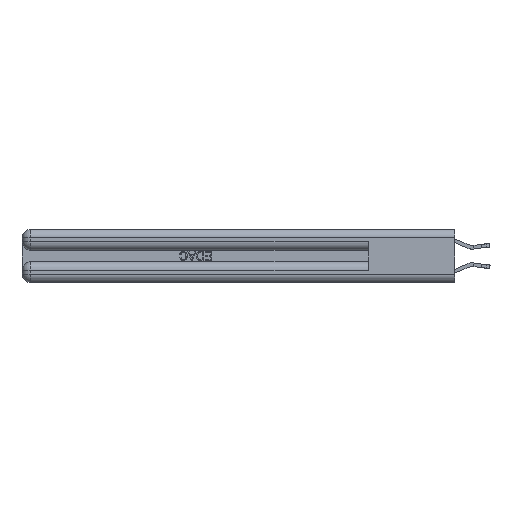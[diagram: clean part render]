
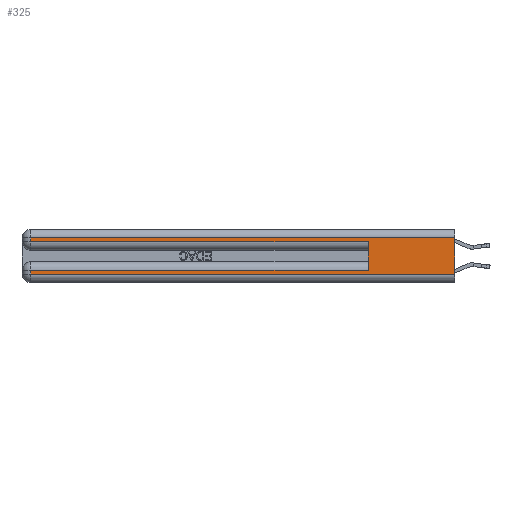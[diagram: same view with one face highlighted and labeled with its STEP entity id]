
A CAD part, left-side view. The second image highlights one B-rep face of the part: STEP entity #325.
In plain terms, the highlighted planar face has unit normal (-1, 0, 0).
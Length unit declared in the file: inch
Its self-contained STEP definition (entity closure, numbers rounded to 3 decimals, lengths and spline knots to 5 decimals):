
#17 = CARTESIAN_POINT ( 'NONE',  ( 0., 2.94, 0.085 ) ) ;
#325 = ADVANCED_FACE ( 'NONE', ( #17375 ), #10696, .F. ) ;
#335 = CARTESIAN_POINT ( 'NONE',  ( 0., 2.94, 0.285 ) ) ;
#1015 = EDGE_LOOP ( 'NONE', ( #27941, #22565, #4123, #26531, #24649, #1185, #6772, #17816 ) ) ;
#1168 = CARTESIAN_POINT ( 'NONE',  ( 0., 2.94, 0.37 ) ) ;
#1185 = ORIENTED_EDGE ( 'NONE', *, *, #25281, .T. ) ;
#1604 = CARTESIAN_POINT ( 'NONE',  ( 0., 0., 0.06 ) ) ;
#1729 = CARTESIAN_POINT ( 'NONE',  ( 0., 0., 0.31 ) ) ;
#3214 = EDGE_CURVE ( 'NONE', #27046, #27026, #27823, .T. ) ;
#4123 = ORIENTED_EDGE ( 'NONE', *, *, #29587, .T. ) ;
#4494 = VERTEX_POINT ( 'NONE', #27971 ) ;
#5132 = VECTOR ( 'NONE', #17609, 39.37008 ) ;
#5583 = EDGE_CURVE ( 'NONE', #21822, #4494, #6006, .T. ) ;
#6006 = LINE ( 'NONE', #1729, #16646 ) ;
#6173 = CARTESIAN_POINT ( 'NONE',  ( 0., 0., 0.285 ) ) ;
#6772 = ORIENTED_EDGE ( 'NONE', *, *, #12108, .T. ) ;
#7667 = LINE ( 'NONE', #13862, #24951 ) ;
#8050 = VECTOR ( 'NONE', #26826, 39.37008 ) ;
#8410 = DIRECTION ( 'NONE',  ( 1., 0., 0. ) ) ;
#8516 = CARTESIAN_POINT ( 'NONE',  ( 0., 0., 0.37 ) ) ;
#8801 = LINE ( 'NONE', #1168, #5132 ) ;
#8876 = DIRECTION ( 'NONE',  ( 0., -1., 0. ) ) ;
#8949 = VERTEX_POINT ( 'NONE', #23475 ) ;
#9177 = CARTESIAN_POINT ( 'NONE',  ( 0., 0.6, 0.145 ) ) ;
#10412 = CARTESIAN_POINT ( 'NONE',  ( 0., 0., 0.085 ) ) ;
#10696 = PLANE ( 'NONE',  #25810 ) ;
#11156 = VECTOR ( 'NONE', #14188, 39.37008 ) ;
#12108 = EDGE_CURVE ( 'NONE', #26962, #8949, #8801, .T. ) ;
#12229 = CARTESIAN_POINT ( 'NONE',  ( 0., 0., 0.31 ) ) ;
#12428 = EDGE_CURVE ( 'NONE', #21822, #18308, #7667, .T. ) ;
#13729 = DIRECTION ( 'NONE',  ( 0., 1., 0. ) ) ;
#13862 = CARTESIAN_POINT ( 'NONE',  ( 0., 0., 0.37 ) ) ;
#14188 = DIRECTION ( 'NONE',  ( 0., 0., 1. ) ) ;
#14235 = VECTOR ( 'NONE', #27121, 39.37008 ) ;
#15751 = DIRECTION ( 'NONE',  ( 0., 0., -1. ) ) ;
#16646 = VECTOR ( 'NONE', #13729, 39.37008 ) ;
#17375 = FACE_OUTER_BOUND ( 'NONE', #1015, .T. ) ;
#17609 = DIRECTION ( 'NONE',  ( 0., 0., -1. ) ) ;
#17816 = ORIENTED_EDGE ( 'NONE', *, *, #19616, .T. ) ;
#17860 = CARTESIAN_POINT ( 'NONE',  ( 0., 0.6, 0.085 ) ) ;
#18063 = EDGE_CURVE ( 'NONE', #24767, #27026, #29871, .T. ) ;
#18308 = VERTEX_POINT ( 'NONE', #20994 ) ;
#18718 = LINE ( 'NONE', #1604, #28209 ) ;
#19019 = VECTOR ( 'NONE', #15751, 39.37008 ) ;
#19130 = LINE ( 'NONE', #10412, #8050 ) ;
#19399 = LINE ( 'NONE', #20140, #19019 ) ;
#19616 = EDGE_CURVE ( 'NONE', #8949, #18308, #18718, .T. ) ;
#19984 = DIRECTION ( 'NONE',  ( 0., 0., -1. ) ) ;
#20140 = CARTESIAN_POINT ( 'NONE',  ( 0., 2.94, 0.37 ) ) ;
#20994 = CARTESIAN_POINT ( 'NONE',  ( 0., 0., 0.06 ) ) ;
#21669 = CARTESIAN_POINT ( 'NONE',  ( 0., 0.6, 0.285 ) ) ;
#21822 = VERTEX_POINT ( 'NONE', #12229 ) ;
#22565 = ORIENTED_EDGE ( 'NONE', *, *, #5583, .T. ) ;
#23475 = CARTESIAN_POINT ( 'NONE',  ( 0., 2.94, 0.06 ) ) ;
#24649 = ORIENTED_EDGE ( 'NONE', *, *, #18063, .F. ) ;
#24767 = VERTEX_POINT ( 'NONE', #17860 ) ;
#24951 = VECTOR ( 'NONE', #27838, 39.37008 ) ;
#25281 = EDGE_CURVE ( 'NONE', #24767, #26962, #19130, .T. ) ;
#25810 = AXIS2_PLACEMENT_3D ( 'NONE', #8516, #8410, #19984 ) ;
#26531 = ORIENTED_EDGE ( 'NONE', *, *, #3214, .T. ) ;
#26826 = DIRECTION ( 'NONE',  ( 0., 1., 0. ) ) ;
#26962 = VERTEX_POINT ( 'NONE', #17 ) ;
#27026 = VERTEX_POINT ( 'NONE', #21669 ) ;
#27046 = VERTEX_POINT ( 'NONE', #335 ) ;
#27121 = DIRECTION ( 'NONE',  ( 0., -1., 0. ) ) ;
#27823 = LINE ( 'NONE', #6173, #14235 ) ;
#27838 = DIRECTION ( 'NONE',  ( 0., 0., -1. ) ) ;
#27941 = ORIENTED_EDGE ( 'NONE', *, *, #12428, .F. ) ;
#27971 = CARTESIAN_POINT ( 'NONE',  ( 0., 2.94, 0.31 ) ) ;
#28209 = VECTOR ( 'NONE', #8876, 39.37008 ) ;
#29587 = EDGE_CURVE ( 'NONE', #4494, #27046, #19399, .T. ) ;
#29871 = LINE ( 'NONE', #9177, #11156 ) ;
